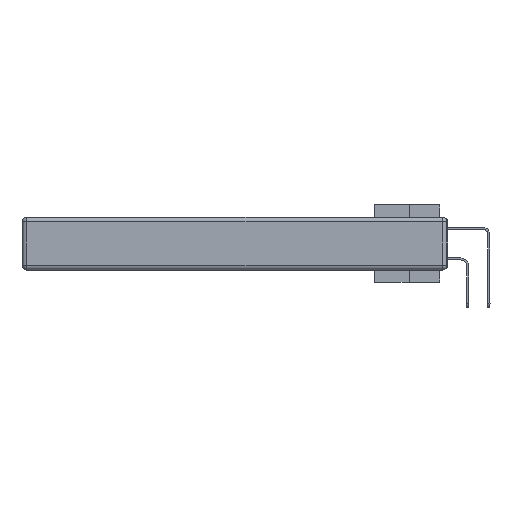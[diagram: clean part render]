
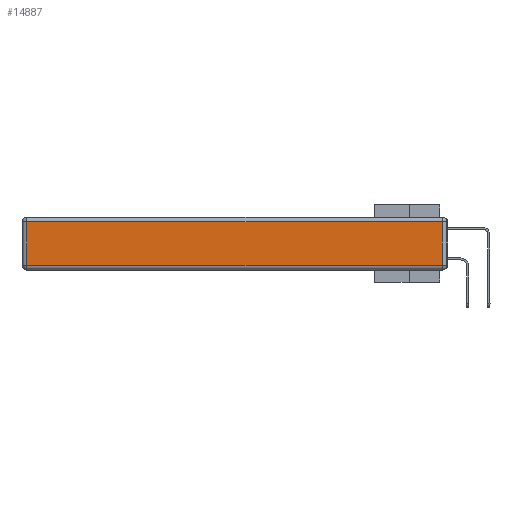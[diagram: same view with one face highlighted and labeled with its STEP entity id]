
A CAD part, left-side view. The second image highlights one B-rep face of the part: STEP entity #14887.
In plain terms, the highlighted planar face has unit normal (-1, 0, 0).
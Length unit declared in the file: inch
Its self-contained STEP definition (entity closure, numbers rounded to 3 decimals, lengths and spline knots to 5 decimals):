
#1718 = ORIENTED_EDGE ( 'NONE', *, *, #30751, .T. ) ;
#2358 = CARTESIAN_POINT ( 'NONE',  ( 0., 2.72, -0.313 ) ) ;
#2414 = EDGE_CURVE ( 'NONE', #9556, #23394, #15959, .T. ) ;
#4574 = CARTESIAN_POINT ( 'NONE',  ( 0., 2.72, -0.343 ) ) ;
#4996 = FACE_OUTER_BOUND ( 'NONE', #12085, .T. ) ;
#5288 = LINE ( 'NONE', #12981, #30330 ) ;
#7660 = DIRECTION ( 'NONE',  ( -1., 0., 0. ) ) ;
#8061 = AXIS2_PLACEMENT_3D ( 'NONE', #20423, #7660, #25481 ) ;
#8421 = CARTESIAN_POINT ( 'NONE',  ( 0., 0., -0.313 ) ) ;
#9556 = VERTEX_POINT ( 'NONE', #13050 ) ;
#12085 = EDGE_LOOP ( 'NONE', ( #1718, #18414, #16883, #13628 ) ) ;
#12981 = CARTESIAN_POINT ( 'NONE',  ( 0., 2.75, -0.03 ) ) ;
#13050 = CARTESIAN_POINT ( 'NONE',  ( 0., 0.03, -0.313 ) ) ;
#13628 = ORIENTED_EDGE ( 'NONE', *, *, #26509, .T. ) ;
#14803 = DIRECTION ( 'NONE',  ( 0., 0., -1. ) ) ;
#14887 = ADVANCED_FACE ( 'NONE', ( #4996 ), #15217, .T. ) ;
#15217 = PLANE ( 'NONE',  #8061 ) ;
#15514 = DIRECTION ( 'NONE',  ( 0., 1., 0. ) ) ;
#15959 = LINE ( 'NONE', #18479, #26866 ) ;
#16128 = VERTEX_POINT ( 'NONE', #2358 ) ;
#16883 = ORIENTED_EDGE ( 'NONE', *, *, #32213, .T. ) ;
#17038 = CARTESIAN_POINT ( 'NONE',  ( 0., 0.03, -0.03 ) ) ;
#18170 = LINE ( 'NONE', #8421, #25941 ) ;
#18414 = ORIENTED_EDGE ( 'NONE', *, *, #2414, .T. ) ;
#18479 = CARTESIAN_POINT ( 'NONE',  ( 0., 0.03, -0.343 ) ) ;
#18974 = DIRECTION ( 'NONE',  ( 0., 0., 1. ) ) ;
#19683 = LINE ( 'NONE', #4574, #25798 ) ;
#20423 = CARTESIAN_POINT ( 'NONE',  ( 0., 0., -0.343 ) ) ;
#23199 = DIRECTION ( 'NONE',  ( 0., -1., 0. ) ) ;
#23394 = VERTEX_POINT ( 'NONE', #17038 ) ;
#25481 = DIRECTION ( 'NONE',  ( 0., 0., 1. ) ) ;
#25798 = VECTOR ( 'NONE', #14803, 39.37008 ) ;
#25941 = VECTOR ( 'NONE', #23199, 39.37008 ) ;
#26509 = EDGE_CURVE ( 'NONE', #29386, #16128, #19683, .T. ) ;
#26866 = VECTOR ( 'NONE', #18974, 39.37008 ) ;
#28078 = CARTESIAN_POINT ( 'NONE',  ( 0., 2.72, -0.03 ) ) ;
#29386 = VERTEX_POINT ( 'NONE', #28078 ) ;
#30330 = VECTOR ( 'NONE', #15514, 39.37008 ) ;
#30751 = EDGE_CURVE ( 'NONE', #16128, #9556, #18170, .T. ) ;
#32213 = EDGE_CURVE ( 'NONE', #23394, #29386, #5288, .T. ) ;
